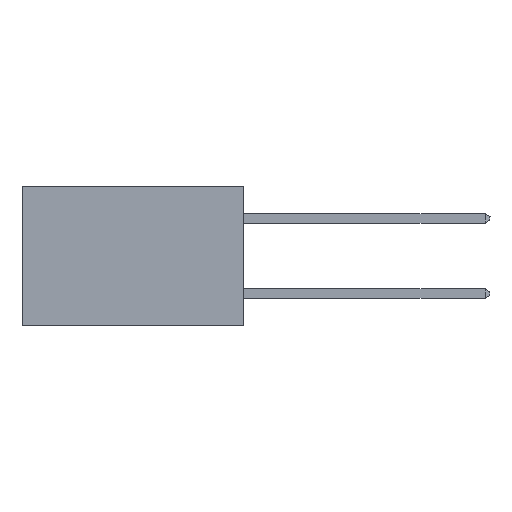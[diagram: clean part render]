
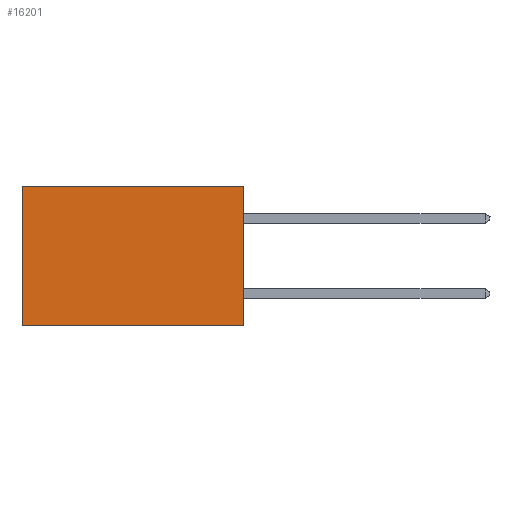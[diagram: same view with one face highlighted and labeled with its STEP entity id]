
A CAD part, left-side view. The second image highlights one B-rep face of the part: STEP entity #16201.
In plain terms, the highlighted planar face has unit normal (-1, 0, 0).
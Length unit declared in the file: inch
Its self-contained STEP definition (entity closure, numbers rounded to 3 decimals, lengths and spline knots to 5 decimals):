
#1087 = CARTESIAN_POINT ( 'NONE',  ( 0.277, 0., -0.37 ) ) ;
#1340 = CARTESIAN_POINT ( 'NONE',  ( 0.277, 0., -0.37 ) ) ;
#1504 = EDGE_CURVE ( 'NONE', #23288, #4042, #2511, .T. ) ;
#2511 = LINE ( 'NONE', #6235, #7401 ) ;
#2902 = DIRECTION ( 'NONE',  ( 1., 0., 0. ) ) ;
#2967 = CARTESIAN_POINT ( 'NONE',  ( 0.277, 0., 0. ) ) ;
#3860 = VECTOR ( 'NONE', #20252, 39.37008 ) ;
#4042 = VERTEX_POINT ( 'NONE', #16570 ) ;
#5066 = ORIENTED_EDGE ( 'NONE', *, *, #1504, .T. ) ;
#5919 = EDGE_CURVE ( 'NONE', #6126, #4042, #18453, .T. ) ;
#5922 = FACE_OUTER_BOUND ( 'NONE', #21519, .T. ) ;
#6126 = VERTEX_POINT ( 'NONE', #18568 ) ;
#6235 = CARTESIAN_POINT ( 'NONE',  ( 0.277, 0.59, -0.37 ) ) ;
#6766 = DIRECTION ( 'NONE',  ( 0., 0., -1. ) ) ;
#7401 = VECTOR ( 'NONE', #18282, 39.37008 ) ;
#8419 = CARTESIAN_POINT ( 'NONE',  ( 0.277, 0., 0. ) ) ;
#8789 = VECTOR ( 'NONE', #10289, 39.37008 ) ;
#8947 = EDGE_CURVE ( 'NONE', #11592, #6126, #22274, .T. ) ;
#9701 = ORIENTED_EDGE ( 'NONE', *, *, #5919, .F. ) ;
#10289 = DIRECTION ( 'NONE',  ( 0., 1., 0. ) ) ;
#11141 = ORIENTED_EDGE ( 'NONE', *, *, #8947, .F. ) ;
#11592 = VERTEX_POINT ( 'NONE', #2967 ) ;
#12077 = PLANE ( 'NONE',  #17363 ) ;
#12678 = VECTOR ( 'NONE', #6766, 39.37008 ) ;
#15746 = DIRECTION ( 'NONE',  ( 0., 0., -1. ) ) ;
#16201 = ADVANCED_FACE ( 'NONE', ( #5922 ), #12077, .F. ) ;
#16570 = CARTESIAN_POINT ( 'NONE',  ( 0.277, 0.59, -0.37 ) ) ;
#16940 = EDGE_CURVE ( 'NONE', #11592, #23288, #18460, .T. ) ;
#17363 = AXIS2_PLACEMENT_3D ( 'NONE', #1087, #2902, #15746 ) ;
#18282 = DIRECTION ( 'NONE',  ( 0., 0., -1. ) ) ;
#18336 = ORIENTED_EDGE ( 'NONE', *, *, #16940, .T. ) ;
#18397 = CARTESIAN_POINT ( 'NONE',  ( 0.277, 0.59, 0. ) ) ;
#18453 = LINE ( 'NONE', #20273, #3860 ) ;
#18460 = LINE ( 'NONE', #8419, #8789 ) ;
#18568 = CARTESIAN_POINT ( 'NONE',  ( 0.277, 0., -0.37 ) ) ;
#20252 = DIRECTION ( 'NONE',  ( 0., 1., 0. ) ) ;
#20273 = CARTESIAN_POINT ( 'NONE',  ( 0.277, 0., -0.37 ) ) ;
#21519 = EDGE_LOOP ( 'NONE', ( #5066, #9701, #11141, #18336 ) ) ;
#22274 = LINE ( 'NONE', #1340, #12678 ) ;
#23288 = VERTEX_POINT ( 'NONE', #18397 ) ;
